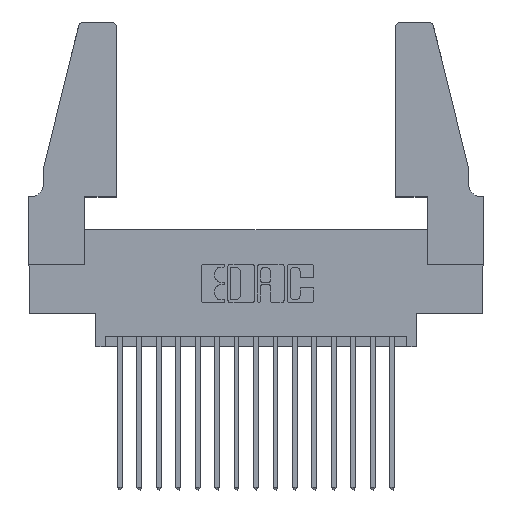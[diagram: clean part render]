
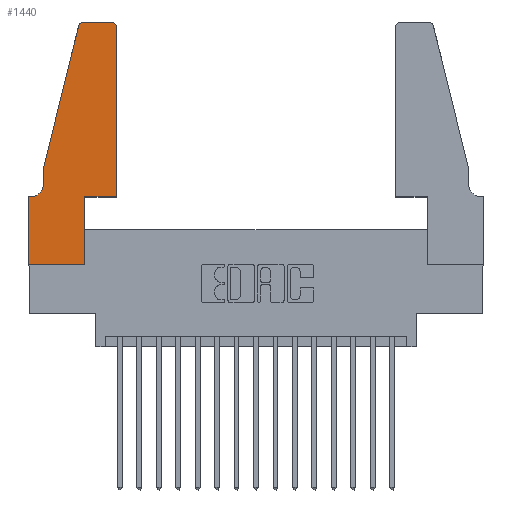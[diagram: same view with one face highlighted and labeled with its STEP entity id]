
A CAD part, top view. The second image highlights one B-rep face of the part: STEP entity #1440.
In plain terms, the highlighted planar face has unit normal (0, 0, 1).
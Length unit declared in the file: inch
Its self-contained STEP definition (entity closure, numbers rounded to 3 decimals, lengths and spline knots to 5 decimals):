
#20 = EDGE_CURVE ( 'NONE', #16477, #5685, #11385, .T. ) ;
#30 = DIRECTION ( 'NONE',  ( 0., 0., -1. ) ) ;
#325 = FACE_OUTER_BOUND ( 'NONE', #873, .T. ) ;
#873 = EDGE_LOOP ( 'NONE', ( #883, #1448, #12159, #10001, #13285, #17313, #8923, #6657, #17543, #13420, #6499, #12975 ) ) ;
#883 = ORIENTED_EDGE ( 'NONE', *, *, #11249, .T. ) ;
#961 = DIRECTION ( 'NONE',  ( 1., 0., 0. ) ) ;
#974 = CARTESIAN_POINT ( 'NONE',  ( 0.4205, 1.25, 0.37 ) ) ;
#1440 = ADVANCED_FACE ( 'NONE', ( #325 ), #16240, .T. ) ;
#1448 = ORIENTED_EDGE ( 'NONE', *, *, #8293, .T. ) ;
#1582 = EDGE_CURVE ( 'NONE', #10392, #16477, #12822, .T. ) ;
#2003 = VERTEX_POINT ( 'NONE', #15311 ) ;
#2085 = CARTESIAN_POINT ( 'NONE',  ( 0., 0., 0.37 ) ) ;
#2666 = VECTOR ( 'NONE', #6036, 39.37008 ) ;
#2816 = EDGE_CURVE ( 'NONE', #3834, #11438, #11709, .T. ) ;
#3151 = VECTOR ( 'NONE', #5537, 39.37008 ) ;
#3289 = LINE ( 'NONE', #8181, #16419 ) ;
#3372 = CARTESIAN_POINT ( 'NONE',  ( 0.284, 1.22, 0.37 ) ) ;
#3539 = VECTOR ( 'NONE', #12991, 39.37008 ) ;
#3834 = VERTEX_POINT ( 'NONE', #4395 ) ;
#3884 = DIRECTION ( 'NONE',  ( 1., 0., 0. ) ) ;
#4130 = DIRECTION ( 'NONE',  ( 0., 1., 0. ) ) ;
#4395 = CARTESIAN_POINT ( 'NONE',  ( 0.4505, 1.22, 0.37 ) ) ;
#4456 = CARTESIAN_POINT ( 'NONE',  ( 0., 0., 0.37 ) ) ;
#4677 = CARTESIAN_POINT ( 'NONE',  ( 0., 0., 0.37 ) ) ;
#4798 = DIRECTION ( 'NONE',  ( 1., 0., 0. ) ) ;
#5218 = VERTEX_POINT ( 'NONE', #7431 ) ;
#5537 = DIRECTION ( 'NONE',  ( -0.239, -0.971, 0. ) ) ;
#5656 = VECTOR ( 'NONE', #11817, 39.37008 ) ;
#5685 = VERTEX_POINT ( 'NONE', #13724 ) ;
#6036 = DIRECTION ( 'NONE',  ( 0., -1., 0. ) ) ;
#6347 = CARTESIAN_POINT ( 'NONE',  ( 0., 0.35, 0.37 ) ) ;
#6420 = DIRECTION ( 'NONE',  ( 0., 0., 1. ) ) ;
#6499 = ORIENTED_EDGE ( 'NONE', *, *, #11535, .T. ) ;
#6657 = ORIENTED_EDGE ( 'NONE', *, *, #15419, .T. ) ;
#6753 = DIRECTION ( 'NONE',  ( 0., -1., 0. ) ) ;
#6971 = EDGE_CURVE ( 'NONE', #2003, #17133, #16696, .T. ) ;
#7110 = LINE ( 'NONE', #14806, #10255 ) ;
#7139 = VECTOR ( 'NONE', #14693, 39.37008 ) ;
#7389 = VECTOR ( 'NONE', #961, 39.37008 ) ;
#7431 = CARTESIAN_POINT ( 'NONE',  ( 0.25487, 1.22718, 0.37 ) ) ;
#7619 = AXIS2_PLACEMENT_3D ( 'NONE', #8351, #30, #9715 ) ;
#7865 = VERTEX_POINT ( 'NONE', #14623 ) ;
#7986 = CARTESIAN_POINT ( 'NONE',  ( 0.0755, 0.35, 0.37 ) ) ;
#8181 = CARTESIAN_POINT ( 'NONE',  ( 0.4505, 0.35, 0.37 ) ) ;
#8293 = EDGE_CURVE ( 'NONE', #13976, #5218, #13488, .T. ) ;
#8351 = CARTESIAN_POINT ( 'NONE',  ( 0.0055, 0.42, 0.37 ) ) ;
#8781 = CARTESIAN_POINT ( 'NONE',  ( 0.4505, 0.35, 0.37 ) ) ;
#8923 = ORIENTED_EDGE ( 'NONE', *, *, #16590, .T. ) ;
#8988 = DIRECTION ( 'NONE',  ( 1., 0., 0. ) ) ;
#9117 = VERTEX_POINT ( 'NONE', #6347 ) ;
#9543 = AXIS2_PLACEMENT_3D ( 'NONE', #3372, #12874, #4798 ) ;
#9715 = DIRECTION ( 'NONE',  ( -1., 0., 0. ) ) ;
#9976 = LINE ( 'NONE', #17652, #3151 ) ;
#10001 = ORIENTED_EDGE ( 'NONE', *, *, #13753, .T. ) ;
#10255 = VECTOR ( 'NONE', #6753, 39.37008 ) ;
#10358 = LINE ( 'NONE', #4677, #2666 ) ;
#10392 = VERTEX_POINT ( 'NONE', #13274 ) ;
#10462 = CARTESIAN_POINT ( 'NONE',  ( 0.2865, 0.35, 0.37 ) ) ;
#11249 = EDGE_CURVE ( 'NONE', #11438, #13976, #17489, .T. ) ;
#11256 = AXIS2_PLACEMENT_3D ( 'NONE', #17049, #17067, #3884 ) ;
#11385 = LINE ( 'NONE', #8781, #7389 ) ;
#11438 = VERTEX_POINT ( 'NONE', #974 ) ;
#11535 = EDGE_CURVE ( 'NONE', #5685, #3834, #3289, .T. ) ;
#11709 = CIRCLE ( 'NONE', #13540, 0.03 ) ;
#11817 = DIRECTION ( 'NONE',  ( 0., 1., 0. ) ) ;
#12137 = EDGE_CURVE ( 'NONE', #17133, #9117, #14696, .T. ) ;
#12159 = ORIENTED_EDGE ( 'NONE', *, *, #15673, .T. ) ;
#12598 = CARTESIAN_POINT ( 'NONE',  ( 0.284, 1.25, 0.37 ) ) ;
#12822 = LINE ( 'NONE', #10462, #5656 ) ;
#12874 = DIRECTION ( 'NONE',  ( 0., 0., 1. ) ) ;
#12975 = ORIENTED_EDGE ( 'NONE', *, *, #2816, .T. ) ;
#12991 = DIRECTION ( 'NONE',  ( -1., 0., 0. ) ) ;
#13274 = CARTESIAN_POINT ( 'NONE',  ( 0.2865, 0., 0.37 ) ) ;
#13285 = ORIENTED_EDGE ( 'NONE', *, *, #6971, .T. ) ;
#13420 = ORIENTED_EDGE ( 'NONE', *, *, #20, .T. ) ;
#13488 = CIRCLE ( 'NONE', #9543, 0.03 ) ;
#13540 = AXIS2_PLACEMENT_3D ( 'NONE', #14477, #6420, #15826 ) ;
#13724 = CARTESIAN_POINT ( 'NONE',  ( 0.4505, 0.35, 0.37 ) ) ;
#13753 = EDGE_CURVE ( 'NONE', #7865, #2003, #7110, .T. ) ;
#13976 = VERTEX_POINT ( 'NONE', #12598 ) ;
#14195 = VECTOR ( 'NONE', #8988, 39.37008 ) ;
#14477 = CARTESIAN_POINT ( 'NONE',  ( 0.4205, 1.22, 0.37 ) ) ;
#14623 = CARTESIAN_POINT ( 'NONE',  ( 0.0755, 0.5, 0.37 ) ) ;
#14693 = DIRECTION ( 'NONE',  ( -1., 0., 0. ) ) ;
#14696 = LINE ( 'NONE', #7986, #7139 ) ;
#14806 = CARTESIAN_POINT ( 'NONE',  ( 0.0755, 0.5, 0.37 ) ) ;
#15028 = LINE ( 'NONE', #2085, #14195 ) ;
#15058 = CARTESIAN_POINT ( 'NONE',  ( 0.0055, 0.35, 0.37 ) ) ;
#15125 = CARTESIAN_POINT ( 'NONE',  ( 0.2865, 0.35, 0.37 ) ) ;
#15311 = CARTESIAN_POINT ( 'NONE',  ( 0.0755, 0.42, 0.37 ) ) ;
#15419 = EDGE_CURVE ( 'NONE', #15789, #10392, #15028, .T. ) ;
#15662 = CARTESIAN_POINT ( 'NONE',  ( 0.2605, 1.25, 0.37 ) ) ;
#15673 = EDGE_CURVE ( 'NONE', #5218, #7865, #9976, .T. ) ;
#15789 = VERTEX_POINT ( 'NONE', #4456 ) ;
#15826 = DIRECTION ( 'NONE',  ( 1., 0., 0. ) ) ;
#16240 = PLANE ( 'NONE',  #11256 ) ;
#16419 = VECTOR ( 'NONE', #4130, 39.37008 ) ;
#16477 = VERTEX_POINT ( 'NONE', #15125 ) ;
#16590 = EDGE_CURVE ( 'NONE', #9117, #15789, #10358, .T. ) ;
#16696 = CIRCLE ( 'NONE', #7619, 0.07 ) ;
#17049 = CARTESIAN_POINT ( 'NONE',  ( 0., 0.35, 0.37 ) ) ;
#17067 = DIRECTION ( 'NONE',  ( 0., 0., 1. ) ) ;
#17133 = VERTEX_POINT ( 'NONE', #15058 ) ;
#17313 = ORIENTED_EDGE ( 'NONE', *, *, #12137, .T. ) ;
#17489 = LINE ( 'NONE', #15662, #3539 ) ;
#17543 = ORIENTED_EDGE ( 'NONE', *, *, #1582, .T. ) ;
#17652 = CARTESIAN_POINT ( 'NONE',  ( 0.0755, 0.5, 0.37 ) ) ;
